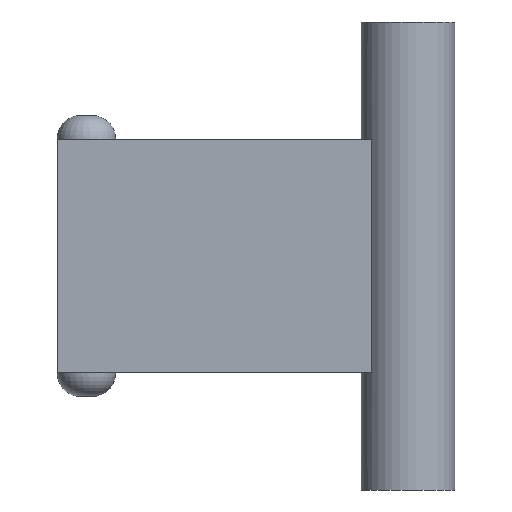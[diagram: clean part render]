
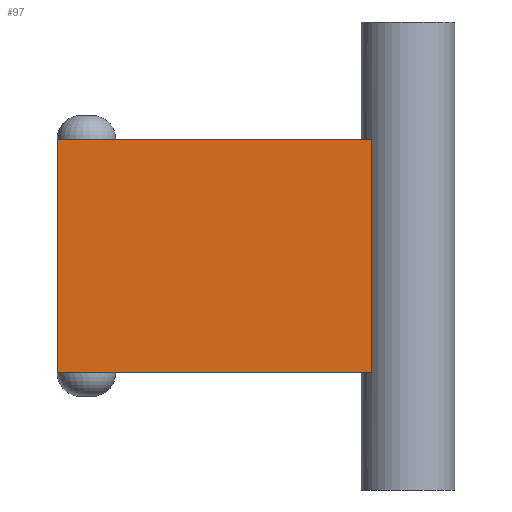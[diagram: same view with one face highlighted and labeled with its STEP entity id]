
A CAD part, front view. The second image highlights one B-rep face of the part: STEP entity #97.
In plain terms, the highlighted planar face has unit normal (0, -1, 0).
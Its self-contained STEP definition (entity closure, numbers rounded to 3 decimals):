
#4 = VERTEX_POINT ( 'NONE', #529 ) ;
#5 = CARTESIAN_POINT ( 'NONE',  ( 11.878, 0., -20. ) ) ;
#28 = AXIS2_PLACEMENT_3D ( 'NONE', #512, #450, #448 ) ;
#44 = DIRECTION ( 'NONE',  ( -1., 0., 0. ) ) ;
#45 = CARTESIAN_POINT ( 'NONE',  ( -15., 0., -10. ) ) ;
#57 = DIRECTION ( 'NONE',  ( -1., 0., 0. ) ) ;
#59 = EDGE_CURVE ( 'NONE', #570, #486, #347, .T. ) ;
#86 = ORIENTED_EDGE ( 'NONE', *, *, #59, .F. ) ;
#97 = ADVANCED_FACE ( 'NONE', ( #337 ), #454, .T. ) ;
#122 = CARTESIAN_POINT ( 'NONE',  ( -15., 0., 10. ) ) ;
#131 = VERTEX_POINT ( 'NONE', #443 ) ;
#143 = ORIENTED_EDGE ( 'NONE', *, *, #343, .F. ) ;
#152 = CARTESIAN_POINT ( 'NONE',  ( 11.878, 0., -10. ) ) ;
#160 = CARTESIAN_POINT ( 'NONE',  ( -15., 0., -10. ) ) ;
#173 = VECTOR ( 'NONE', #505, 1000. ) ;
#204 = ORIENTED_EDGE ( 'NONE', *, *, #305, .F. ) ;
#257 = VERTEX_POINT ( 'NONE', #160 ) ;
#262 = LINE ( 'NONE', #314, #535 ) ;
#268 = VECTOR ( 'NONE', #350, 1000. ) ;
#304 = DIRECTION ( 'NONE',  ( 1., 0., 0. ) ) ;
#305 = EDGE_CURVE ( 'NONE', #4, #570, #520, .T. ) ;
#306 = CARTESIAN_POINT ( 'NONE',  ( -15., 0., 10. ) ) ;
#314 = CARTESIAN_POINT ( 'NONE',  ( -15., 0., 10. ) ) ;
#317 = CARTESIAN_POINT ( 'NONE',  ( -12.5, 0., -10. ) ) ;
#337 = FACE_OUTER_BOUND ( 'NONE', #432, .T. ) ;
#343 = EDGE_CURVE ( 'NONE', #486, #475, #542, .T. ) ;
#347 = LINE ( 'NONE', #5, #173 ) ;
#350 = DIRECTION ( 'NONE',  ( 0., 0., 1. ) ) ;
#354 = LINE ( 'NONE', #306, #268 ) ;
#374 = VECTOR ( 'NONE', #57, 1000. ) ;
#409 = ORIENTED_EDGE ( 'NONE', *, *, #428, .F. ) ;
#419 = ORIENTED_EDGE ( 'NONE', *, *, #456, .F. ) ;
#424 = ORIENTED_EDGE ( 'NONE', *, *, #532, .F. ) ;
#428 = EDGE_CURVE ( 'NONE', #475, #257, #582, .T. ) ;
#432 = EDGE_LOOP ( 'NONE', ( #204, #424, #419, #409, #143, #86 ) ) ;
#438 = CARTESIAN_POINT ( 'NONE',  ( 11.878, 0., 10. ) ) ;
#443 = CARTESIAN_POINT ( 'NONE',  ( -15., 0., 10. ) ) ;
#448 = DIRECTION ( 'NONE',  ( 0., 0., -1. ) ) ;
#450 = DIRECTION ( 'NONE',  ( 0., -1., 0. ) ) ;
#454 = PLANE ( 'NONE',  #28 ) ;
#456 = EDGE_CURVE ( 'NONE', #257, #131, #354, .T. ) ;
#475 = VERTEX_POINT ( 'NONE', #317 ) ;
#480 = CARTESIAN_POINT ( 'NONE',  ( -15., 0., -10. ) ) ;
#486 = VERTEX_POINT ( 'NONE', #152 ) ;
#499 = DIRECTION ( 'NONE',  ( 1., 0., 0. ) ) ;
#505 = DIRECTION ( 'NONE',  ( 0., 0., -1. ) ) ;
#509 = VECTOR ( 'NONE', #44, 1000. ) ;
#512 = CARTESIAN_POINT ( 'NONE',  ( 0., 0., 0. ) ) ;
#520 = LINE ( 'NONE', #122, #564 ) ;
#529 = CARTESIAN_POINT ( 'NONE',  ( -12.5, 0., 10. ) ) ;
#532 = EDGE_CURVE ( 'NONE', #131, #4, #262, .T. ) ;
#535 = VECTOR ( 'NONE', #499, 1000. ) ;
#542 = LINE ( 'NONE', #45, #509 ) ;
#564 = VECTOR ( 'NONE', #304, 1000. ) ;
#570 = VERTEX_POINT ( 'NONE', #438 ) ;
#582 = LINE ( 'NONE', #480, #374 ) ;
